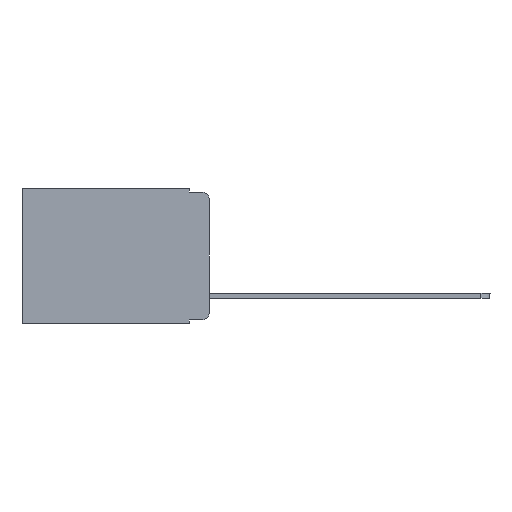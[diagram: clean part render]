
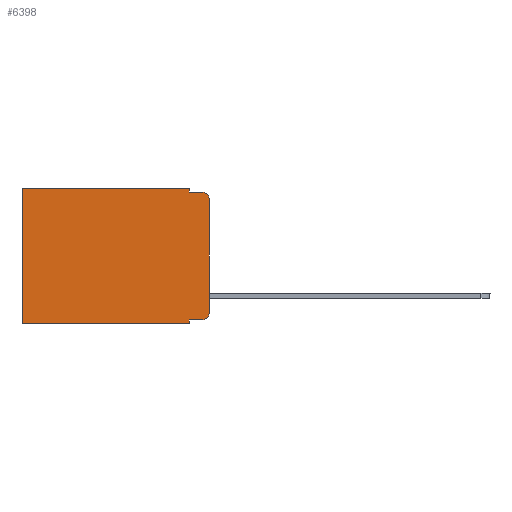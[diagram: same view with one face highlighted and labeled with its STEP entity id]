
A CAD part, left-side view. The second image highlights one B-rep face of the part: STEP entity #6398.
In plain terms, the highlighted planar face has unit normal (-1, 0, 0).
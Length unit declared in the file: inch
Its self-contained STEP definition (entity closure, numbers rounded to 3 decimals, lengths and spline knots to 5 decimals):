
#90 = VERTEX_POINT ( 'NONE', #11093 ) ;
#152 = VERTEX_POINT ( 'NONE', #9048 ) ;
#322 = VERTEX_POINT ( 'NONE', #13925 ) ;
#645 = LINE ( 'NONE', #8438, #7395 ) ;
#1050 = DIRECTION ( 'NONE',  ( 0., 0., -1. ) ) ;
#1209 = DIRECTION ( 'NONE',  ( 0., -1., 0. ) ) ;
#1348 = CIRCLE ( 'NONE', #9483, 0.02 ) ;
#1483 = DIRECTION ( 'NONE',  ( 0., 0., -1. ) ) ;
#1551 = CARTESIAN_POINT ( 'NONE',  ( 0.298, 0.473, -0.343 ) ) ;
#1738 = DIRECTION ( 'NONE',  ( 0., 1., 0. ) ) ;
#2451 = EDGE_LOOP ( 'NONE', ( #7394, #12489, #7287, #3781, #4389, #7621, #6844, #13204, #4713, #8843 ) ) ;
#2469 = DIRECTION ( 'NONE',  ( 0., 0., -1. ) ) ;
#2872 = LINE ( 'NONE', #9334, #8060 ) ;
#2908 = EDGE_CURVE ( 'NONE', #7268, #8919, #6654, .T. ) ;
#3017 = DIRECTION ( 'NONE',  ( 0., 1., 0. ) ) ;
#3488 = EDGE_CURVE ( 'NONE', #10632, #5754, #12132, .T. ) ;
#3781 = ORIENTED_EDGE ( 'NONE', *, *, #6555, .F. ) ;
#3922 = CARTESIAN_POINT ( 'NONE',  ( 0.298, 0., 0. ) ) ;
#4389 = ORIENTED_EDGE ( 'NONE', *, *, #5505, .T. ) ;
#4584 = DIRECTION ( 'NONE',  ( -1., 0., 0. ) ) ;
#4682 = DIRECTION ( 'NONE',  ( 1., 0., 0. ) ) ;
#4713 = ORIENTED_EDGE ( 'NONE', *, *, #12511, .T. ) ;
#4877 = CARTESIAN_POINT ( 'NONE',  ( 0.298, 0., -0.03 ) ) ;
#4912 = CARTESIAN_POINT ( 'NONE',  ( 0.298, 0.051, -0.333 ) ) ;
#4949 = EDGE_CURVE ( 'NONE', #152, #8863, #8049, .T. ) ;
#5002 = AXIS2_PLACEMENT_3D ( 'NONE', #10148, #4682, #12409 ) ;
#5505 = EDGE_CURVE ( 'NONE', #9678, #152, #11812, .T. ) ;
#5754 = VERTEX_POINT ( 'NONE', #7339 ) ;
#6375 = LINE ( 'NONE', #4912, #13439 ) ;
#6398 = ADVANCED_FACE ( 'NONE', ( #14176 ), #6659, .F. ) ;
#6447 = CARTESIAN_POINT ( 'NONE',  ( 0.298, 0.051, -0.01 ) ) ;
#6555 = EDGE_CURVE ( 'NONE', #9678, #7382, #2872, .T. ) ;
#6654 = LINE ( 'NONE', #9788, #13491 ) ;
#6659 = PLANE ( 'NONE',  #5002 ) ;
#6844 = ORIENTED_EDGE ( 'NONE', *, *, #9871, .F. ) ;
#7199 = CARTESIAN_POINT ( 'NONE',  ( 0.298, 0.051, -0.01 ) ) ;
#7268 = VERTEX_POINT ( 'NONE', #8881 ) ;
#7287 = ORIENTED_EDGE ( 'NONE', *, *, #13861, .F. ) ;
#7339 = CARTESIAN_POINT ( 'NONE',  ( 0.298, 0.02, -0.01 ) ) ;
#7382 = VERTEX_POINT ( 'NONE', #7199 ) ;
#7394 = ORIENTED_EDGE ( 'NONE', *, *, #7532, .F. ) ;
#7395 = VECTOR ( 'NONE', #1738, 39.37008 ) ;
#7428 = VECTOR ( 'NONE', #1209, 39.37008 ) ;
#7532 = EDGE_CURVE ( 'NONE', #10632, #90, #9443, .T. ) ;
#7621 = ORIENTED_EDGE ( 'NONE', *, *, #4949, .T. ) ;
#8049 = LINE ( 'NONE', #10313, #9002 ) ;
#8060 = VECTOR ( 'NONE', #1483, 39.37008 ) ;
#8111 = CARTESIAN_POINT ( 'NONE',  ( 0.298, 0.051, -0.343 ) ) ;
#8271 = DIRECTION ( 'NONE',  ( 0., -1., 0. ) ) ;
#8438 = CARTESIAN_POINT ( 'NONE',  ( 0.298, 0., -0.343 ) ) ;
#8637 = LINE ( 'NONE', #6447, #7428 ) ;
#8720 = VECTOR ( 'NONE', #3017, 39.37008 ) ;
#8843 = ORIENTED_EDGE ( 'NONE', *, *, #12760, .T. ) ;
#8863 = VERTEX_POINT ( 'NONE', #1551 ) ;
#8881 = CARTESIAN_POINT ( 'NONE',  ( 0.298, 0.051, -0.333 ) ) ;
#8919 = VERTEX_POINT ( 'NONE', #8111 ) ;
#9002 = VECTOR ( 'NONE', #13585, 39.37008 ) ;
#9048 = CARTESIAN_POINT ( 'NONE',  ( 0.298, 0.473, 0. ) ) ;
#9334 = CARTESIAN_POINT ( 'NONE',  ( 0.298, 0.051, 0. ) ) ;
#9443 = LINE ( 'NONE', #3922, #10395 ) ;
#9483 = AXIS2_PLACEMENT_3D ( 'NONE', #13431, #12346, #11315 ) ;
#9678 = VERTEX_POINT ( 'NONE', #12376 ) ;
#9788 = CARTESIAN_POINT ( 'NONE',  ( 0.298, 0.051, 0. ) ) ;
#9871 = EDGE_CURVE ( 'NONE', #8919, #8863, #645, .T. ) ;
#10148 = CARTESIAN_POINT ( 'NONE',  ( 0.298, 0., 0. ) ) ;
#10313 = CARTESIAN_POINT ( 'NONE',  ( 0.298, 0.473, 0. ) ) ;
#10395 = VECTOR ( 'NONE', #2469, 39.37008 ) ;
#10632 = VERTEX_POINT ( 'NONE', #4877 ) ;
#11093 = CARTESIAN_POINT ( 'NONE',  ( 0.298, 0., -0.313 ) ) ;
#11315 = DIRECTION ( 'NONE',  ( 0., 0., -1. ) ) ;
#11812 = LINE ( 'NONE', #12908, #8720 ) ;
#12132 = CIRCLE ( 'NONE', #14002, 0.02 ) ;
#12240 = CARTESIAN_POINT ( 'NONE',  ( 0.298, 0.02, -0.03 ) ) ;
#12346 = DIRECTION ( 'NONE',  ( -1., 0., 0. ) ) ;
#12376 = CARTESIAN_POINT ( 'NONE',  ( 0.298, 0.051, 0. ) ) ;
#12409 = DIRECTION ( 'NONE',  ( 0., 0., -1. ) ) ;
#12489 = ORIENTED_EDGE ( 'NONE', *, *, #3488, .T. ) ;
#12511 = EDGE_CURVE ( 'NONE', #7268, #322, #6375, .T. ) ;
#12760 = EDGE_CURVE ( 'NONE', #322, #90, #1348, .T. ) ;
#12908 = CARTESIAN_POINT ( 'NONE',  ( 0.298, 0., 0. ) ) ;
#13204 = ORIENTED_EDGE ( 'NONE', *, *, #2908, .F. ) ;
#13431 = CARTESIAN_POINT ( 'NONE',  ( 0.298, 0.02, -0.313 ) ) ;
#13439 = VECTOR ( 'NONE', #8271, 39.37008 ) ;
#13491 = VECTOR ( 'NONE', #1050, 39.37008 ) ;
#13585 = DIRECTION ( 'NONE',  ( 0., 0., -1. ) ) ;
#13815 = DIRECTION ( 'NONE',  ( 0., 0., -1. ) ) ;
#13861 = EDGE_CURVE ( 'NONE', #7382, #5754, #8637, .T. ) ;
#13925 = CARTESIAN_POINT ( 'NONE',  ( 0.298, 0.02, -0.333 ) ) ;
#14002 = AXIS2_PLACEMENT_3D ( 'NONE', #12240, #4584, #13815 ) ;
#14176 = FACE_OUTER_BOUND ( 'NONE', #2451, .T. ) ;
